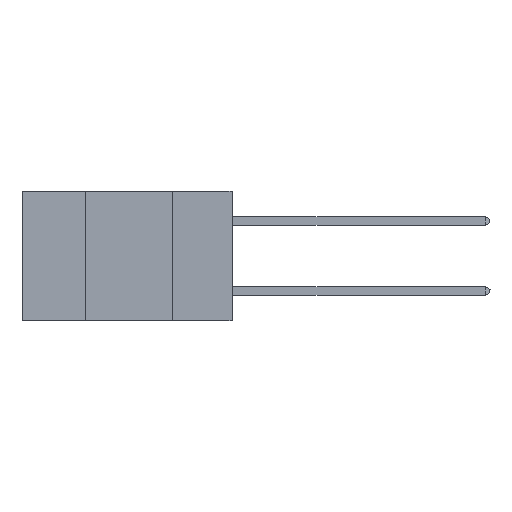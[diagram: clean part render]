
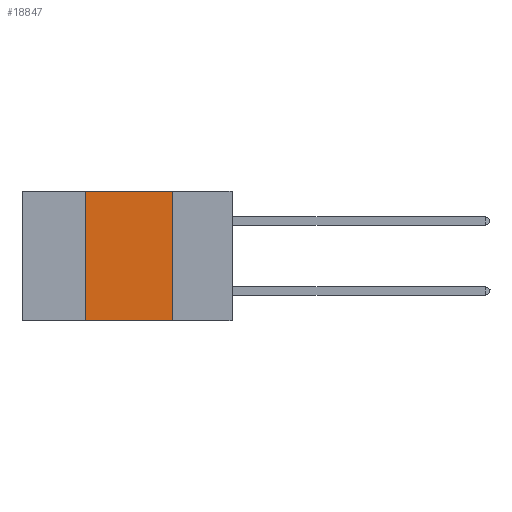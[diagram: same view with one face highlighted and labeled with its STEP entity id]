
A CAD part, left-side view. The second image highlights one B-rep face of the part: STEP entity #18847.
In plain terms, the highlighted planar face has unit normal (-1, 0, 0).
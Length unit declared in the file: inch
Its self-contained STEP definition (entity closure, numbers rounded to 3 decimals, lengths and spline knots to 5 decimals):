
#40 = LINE ( 'NONE', #5178, #8375 ) ;
#53 = EDGE_CURVE ( 'NONE', #16084, #678, #22749, .T. ) ;
#678 = VERTEX_POINT ( 'NONE', #6934 ) ;
#1340 = CARTESIAN_POINT ( 'NONE',  ( 0., 0.42, 0. ) ) ;
#1756 = CARTESIAN_POINT ( 'NONE',  ( 0., 0.6, 0. ) ) ;
#3259 = CARTESIAN_POINT ( 'NONE',  ( 0., 0.17, 0. ) ) ;
#3613 = DIRECTION ( 'NONE',  ( 0., -1., 0. ) ) ;
#4284 = ORIENTED_EDGE ( 'NONE', *, *, #22916, .T. ) ;
#4675 = VERTEX_POINT ( 'NONE', #21394 ) ;
#5178 = CARTESIAN_POINT ( 'NONE',  ( 0., 0.6, -0.37 ) ) ;
#5391 = LINE ( 'NONE', #3259, #24341 ) ;
#6934 = CARTESIAN_POINT ( 'NONE',  ( 0., 0.17, 0. ) ) ;
#7245 = DIRECTION ( 'NONE',  ( 0., 0., -1. ) ) ;
#8375 = VECTOR ( 'NONE', #3613, 39.37008 ) ;
#8499 = EDGE_LOOP ( 'NONE', ( #11457, #15352, #8512, #4284 ) ) ;
#8512 = ORIENTED_EDGE ( 'NONE', *, *, #16083, .F. ) ;
#11251 = FACE_OUTER_BOUND ( 'NONE', #8499, .T. ) ;
#11457 = ORIENTED_EDGE ( 'NONE', *, *, #17852, .F. ) ;
#13340 = DIRECTION ( 'NONE',  ( 0., 0., 1. ) ) ;
#14615 = CARTESIAN_POINT ( 'NONE',  ( 0., 0.42, 0. ) ) ;
#15352 = ORIENTED_EDGE ( 'NONE', *, *, #53, .F. ) ;
#15966 = CARTESIAN_POINT ( 'NONE',  ( 0., 0.6, 0. ) ) ;
#16083 = EDGE_CURVE ( 'NONE', #16107, #16084, #21440, .T. ) ;
#16084 = VERTEX_POINT ( 'NONE', #1340 ) ;
#16107 = VERTEX_POINT ( 'NONE', #17170 ) ;
#17170 = CARTESIAN_POINT ( 'NONE',  ( 0., 0.42, -0.37 ) ) ;
#17322 = VECTOR ( 'NONE', #13340, 39.37008 ) ;
#17815 = PLANE ( 'NONE',  #23339 ) ;
#17852 = EDGE_CURVE ( 'NONE', #678, #4675, #5391, .T. ) ;
#17899 = DIRECTION ( 'NONE',  ( 1., 0., 0. ) ) ;
#18307 = VECTOR ( 'NONE', #20715, 39.37008 ) ;
#18847 = ADVANCED_FACE ( 'NONE', ( #11251 ), #17815, .F. ) ;
#20715 = DIRECTION ( 'NONE',  ( 0., -1., 0. ) ) ;
#21351 = DIRECTION ( 'NONE',  ( 0., 0., -1. ) ) ;
#21394 = CARTESIAN_POINT ( 'NONE',  ( 0., 0.17, -0.37 ) ) ;
#21440 = LINE ( 'NONE', #14615, #17322 ) ;
#22749 = LINE ( 'NONE', #1756, #18307 ) ;
#22916 = EDGE_CURVE ( 'NONE', #16107, #4675, #40, .T. ) ;
#23339 = AXIS2_PLACEMENT_3D ( 'NONE', #15966, #17899, #21351 ) ;
#24341 = VECTOR ( 'NONE', #7245, 39.37008 ) ;
